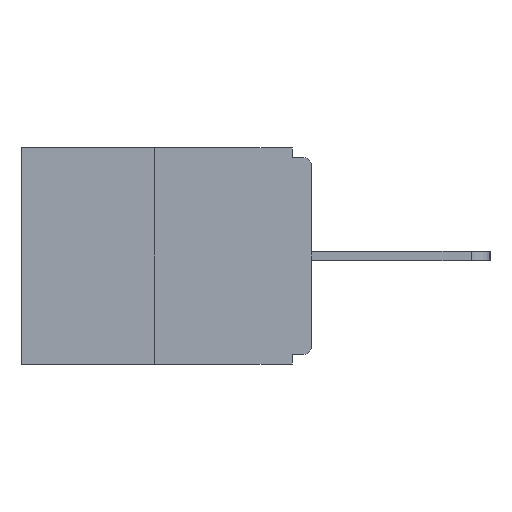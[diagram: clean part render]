
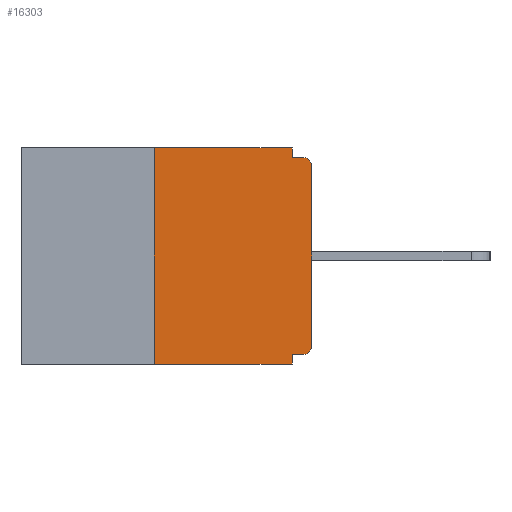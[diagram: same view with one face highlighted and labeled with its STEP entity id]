
A CAD part, left-side view. The second image highlights one B-rep face of the part: STEP entity #16303.
In plain terms, the highlighted planar face has unit normal (-1, 0, 0).
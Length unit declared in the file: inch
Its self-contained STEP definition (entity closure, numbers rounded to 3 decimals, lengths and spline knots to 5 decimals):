
#69 = EDGE_LOOP ( 'NONE', ( #5009, #442, #9621, #13956, #11694, #3909, #3501, #3774, #18818, #12920 ) ) ;
#210 = CARTESIAN_POINT ( 'NONE',  ( 0., 0., 0. ) ) ;
#361 = CARTESIAN_POINT ( 'NONE',  ( 0., 0.25, 0. ) ) ;
#442 = ORIENTED_EDGE ( 'NONE', *, *, #12302, .F. ) ;
#840 = CIRCLE ( 'NONE', #11905, 0.015 ) ;
#1062 = DIRECTION ( 'NONE',  ( 0., 1., 0. ) ) ;
#1078 = LINE ( 'NONE', #3878, #6091 ) ;
#1116 = DIRECTION ( 'NONE',  ( 0., 0., -1. ) ) ;
#1156 = AXIS2_PLACEMENT_3D ( 'NONE', #7096, #5502, #1116 ) ;
#2433 = CARTESIAN_POINT ( 'NONE',  ( 0., 0., -0.015 ) ) ;
#2713 = LINE ( 'NONE', #9079, #10739 ) ;
#3342 = CARTESIAN_POINT ( 'NONE',  ( 0., 0.015, -0.03 ) ) ;
#3501 = ORIENTED_EDGE ( 'NONE', *, *, #15980, .T. ) ;
#3571 = EDGE_CURVE ( 'NONE', #16407, #4836, #6992, .T. ) ;
#3682 = CARTESIAN_POINT ( 'NONE',  ( 0., 0.25, -0.343 ) ) ;
#3709 = CARTESIAN_POINT ( 'NONE',  ( 0., 0.46, -0.343 ) ) ;
#3774 = ORIENTED_EDGE ( 'NONE', *, *, #7219, .T. ) ;
#3852 = VERTEX_POINT ( 'NONE', #3682 ) ;
#3878 = CARTESIAN_POINT ( 'NONE',  ( 0., 0.25, 0. ) ) ;
#3909 = ORIENTED_EDGE ( 'NONE', *, *, #8848, .T. ) ;
#4176 = CARTESIAN_POINT ( 'NONE',  ( 0., 0., -0.03 ) ) ;
#4574 = VECTOR ( 'NONE', #18582, 39.37008 ) ;
#4649 = CIRCLE ( 'NONE', #1156, 0.015 ) ;
#4727 = VECTOR ( 'NONE', #18107, 39.37008 ) ;
#4836 = VERTEX_POINT ( 'NONE', #13779 ) ;
#5009 = ORIENTED_EDGE ( 'NONE', *, *, #10352, .F. ) ;
#5428 = VERTEX_POINT ( 'NONE', #8854 ) ;
#5502 = DIRECTION ( 'NONE',  ( -1., 0., 0. ) ) ;
#5951 = CARTESIAN_POINT ( 'NONE',  ( 0., 0.46, 0. ) ) ;
#6091 = VECTOR ( 'NONE', #8366, 39.37008 ) ;
#6328 = DIRECTION ( 'NONE',  ( 0., 0., -1. ) ) ;
#6992 = LINE ( 'NONE', #13056, #4727 ) ;
#7096 = CARTESIAN_POINT ( 'NONE',  ( 0., 0.015, -0.313 ) ) ;
#7219 = EDGE_CURVE ( 'NONE', #8265, #14085, #840, .T. ) ;
#7356 = VECTOR ( 'NONE', #8797, 39.37008 ) ;
#7798 = EDGE_CURVE ( 'NONE', #3852, #4836, #18613, .T. ) ;
#8265 = VERTEX_POINT ( 'NONE', #4176 ) ;
#8338 = VERTEX_POINT ( 'NONE', #14632 ) ;
#8366 = DIRECTION ( 'NONE',  ( 0., 0., 1. ) ) ;
#8797 = DIRECTION ( 'NONE',  ( 0., 0., -1. ) ) ;
#8848 = EDGE_CURVE ( 'NONE', #5428, #8338, #4649, .T. ) ;
#8854 = CARTESIAN_POINT ( 'NONE',  ( 0., 0.015, -0.328 ) ) ;
#9079 = CARTESIAN_POINT ( 'NONE',  ( 0., 0.46, 0. ) ) ;
#9202 = CARTESIAN_POINT ( 'NONE',  ( 0., 0.031, 0. ) ) ;
#9287 = VECTOR ( 'NONE', #17339, 39.37008 ) ;
#9621 = ORIENTED_EDGE ( 'NONE', *, *, #7798, .T. ) ;
#10352 = EDGE_CURVE ( 'NONE', #18101, #17191, #2713, .T. ) ;
#10739 = VECTOR ( 'NONE', #16622, 39.37008 ) ;
#11694 = ORIENTED_EDGE ( 'NONE', *, *, #17887, .F. ) ;
#11865 = CARTESIAN_POINT ( 'NONE',  ( 0., 0.031, 0. ) ) ;
#11884 = EDGE_CURVE ( 'NONE', #14921, #14085, #16049, .T. ) ;
#11905 = AXIS2_PLACEMENT_3D ( 'NONE', #3342, #13893, #6328 ) ;
#11949 = EDGE_CURVE ( 'NONE', #17191, #14921, #14950, .T. ) ;
#12302 = EDGE_CURVE ( 'NONE', #3852, #18101, #1078, .T. ) ;
#12423 = CARTESIAN_POINT ( 'NONE',  ( 0., 0.031, -0.328 ) ) ;
#12920 = ORIENTED_EDGE ( 'NONE', *, *, #11949, .F. ) ;
#13056 = CARTESIAN_POINT ( 'NONE',  ( 0., 0.031, -0.343 ) ) ;
#13198 = CARTESIAN_POINT ( 'NONE',  ( 0., 0., -0.328 ) ) ;
#13779 = CARTESIAN_POINT ( 'NONE',  ( 0., 0.031, -0.343 ) ) ;
#13829 = LINE ( 'NONE', #210, #4574 ) ;
#13893 = DIRECTION ( 'NONE',  ( -1., 0., 0. ) ) ;
#13956 = ORIENTED_EDGE ( 'NONE', *, *, #3571, .F. ) ;
#14085 = VERTEX_POINT ( 'NONE', #14661 ) ;
#14169 = VECTOR ( 'NONE', #1062, 39.37008 ) ;
#14632 = CARTESIAN_POINT ( 'NONE',  ( 0., 0., -0.313 ) ) ;
#14661 = CARTESIAN_POINT ( 'NONE',  ( 0., 0.015, -0.015 ) ) ;
#14697 = LINE ( 'NONE', #13198, #14169 ) ;
#14921 = VERTEX_POINT ( 'NONE', #17489 ) ;
#14950 = LINE ( 'NONE', #11865, #7356 ) ;
#14994 = FACE_OUTER_BOUND ( 'NONE', #69, .T. ) ;
#15932 = DIRECTION ( 'NONE',  ( 0., -1., 0. ) ) ;
#15980 = EDGE_CURVE ( 'NONE', #8338, #8265, #13829, .T. ) ;
#16049 = LINE ( 'NONE', #2433, #9287 ) ;
#16303 = ADVANCED_FACE ( 'NONE', ( #14994 ), #16680, .F. ) ;
#16407 = VERTEX_POINT ( 'NONE', #12423 ) ;
#16582 = DIRECTION ( 'NONE',  ( 0., 0., -1. ) ) ;
#16622 = DIRECTION ( 'NONE',  ( 0., -1., 0. ) ) ;
#16680 = PLANE ( 'NONE',  #16975 ) ;
#16975 = AXIS2_PLACEMENT_3D ( 'NONE', #5951, #19555, #16582 ) ;
#17191 = VERTEX_POINT ( 'NONE', #9202 ) ;
#17313 = VECTOR ( 'NONE', #15932, 39.37008 ) ;
#17339 = DIRECTION ( 'NONE',  ( 0., -1., 0. ) ) ;
#17489 = CARTESIAN_POINT ( 'NONE',  ( 0., 0.031, -0.015 ) ) ;
#17887 = EDGE_CURVE ( 'NONE', #5428, #16407, #14697, .T. ) ;
#18101 = VERTEX_POINT ( 'NONE', #361 ) ;
#18107 = DIRECTION ( 'NONE',  ( 0., 0., -1. ) ) ;
#18582 = DIRECTION ( 'NONE',  ( 0., 0., 1. ) ) ;
#18613 = LINE ( 'NONE', #3709, #17313 ) ;
#18818 = ORIENTED_EDGE ( 'NONE', *, *, #11884, .F. ) ;
#19555 = DIRECTION ( 'NONE',  ( 1., 0., 0. ) ) ;
